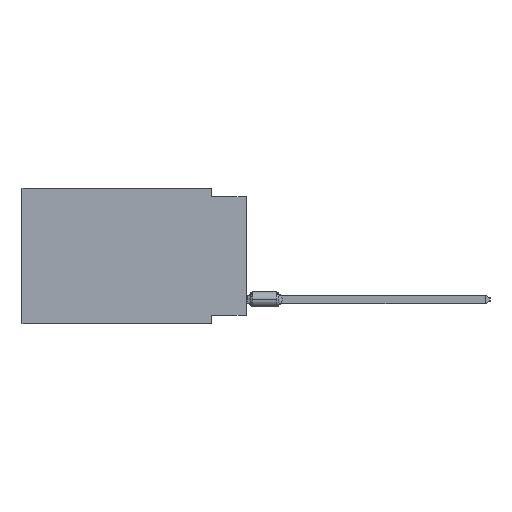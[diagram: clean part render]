
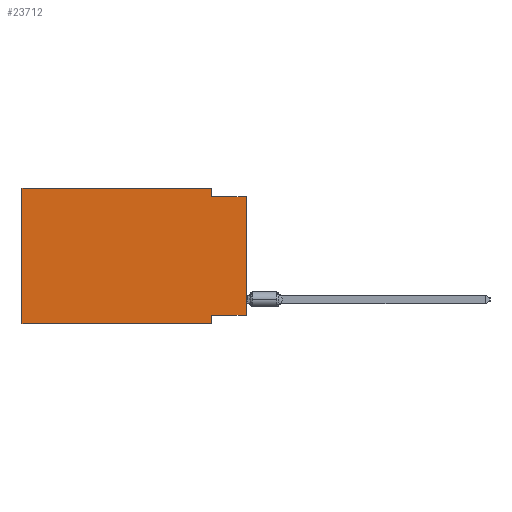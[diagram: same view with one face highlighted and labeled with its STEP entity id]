
A CAD part, left-side view. The second image highlights one B-rep face of the part: STEP entity #23712.
In plain terms, the highlighted planar face has unit normal (-1, 0, 0).
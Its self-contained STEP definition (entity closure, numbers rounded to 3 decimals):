
#1113 = CARTESIAN_POINT ( 'NONE',  ( 0., 16.383, 0. ) ) ;
#2373 = CARTESIAN_POINT ( 'NONE',  ( 0., 2.54, -9.906 ) ) ;
#3141 = VECTOR ( 'NONE', #3512, 1000. ) ;
#3512 = DIRECTION ( 'NONE',  ( 0., 0., -1. ) ) ;
#3820 = CARTESIAN_POINT ( 'NONE',  ( 0., 16.383, 0. ) ) ;
#5066 = ORIENTED_EDGE ( 'NONE', *, *, #47466, .T. ) ;
#7582 = VERTEX_POINT ( 'NONE', #53721 ) ;
#8241 = ORIENTED_EDGE ( 'NONE', *, *, #48617, .F. ) ;
#8436 = VECTOR ( 'NONE', #38168, 1000. ) ;
#9163 = DIRECTION ( 'NONE',  ( 0., 0., -1. ) ) ;
#11869 = VECTOR ( 'NONE', #49822, 1000. ) ;
#12670 = EDGE_CURVE ( 'NONE', #59389, #61183, #68344, .T. ) ;
#13704 = DIRECTION ( 'NONE',  ( 1., 0., 0. ) ) ;
#14302 = CARTESIAN_POINT ( 'NONE',  ( 0., 2.54, -9.906 ) ) ;
#14385 = PLANE ( 'NONE',  #55197 ) ;
#15514 = CARTESIAN_POINT ( 'NONE',  ( 0., 0., -0.635 ) ) ;
#16459 = LINE ( 'NONE', #37714, #11869 ) ;
#16998 = DIRECTION ( 'NONE',  ( 0., -1., 0. ) ) ;
#17649 = VERTEX_POINT ( 'NONE', #27561 ) ;
#18275 = CARTESIAN_POINT ( 'NONE',  ( 0., 16.383, 0. ) ) ;
#19437 = VERTEX_POINT ( 'NONE', #59192 ) ;
#20833 = LINE ( 'NONE', #64769, #36791 ) ;
#22191 = ORIENTED_EDGE ( 'NONE', *, *, #49745, .T. ) ;
#22597 = EDGE_CURVE ( 'NONE', #62183, #17649, #51913, .T. ) ;
#23712 = ADVANCED_FACE ( 'NONE', ( #56230 ), #14385, .F. ) ;
#25051 = DIRECTION ( 'NONE',  ( 0., -1., 0. ) ) ;
#27561 = CARTESIAN_POINT ( 'NONE',  ( 0., 2.54, 0. ) ) ;
#31141 = EDGE_CURVE ( 'NONE', #7582, #59389, #46911, .T. ) ;
#34273 = ORIENTED_EDGE ( 'NONE', *, *, #31141, .F. ) ;
#34578 = EDGE_CURVE ( 'NONE', #19437, #63240, #20833, .T. ) ;
#34847 = VECTOR ( 'NONE', #57052, 1000. ) ;
#35035 = VECTOR ( 'NONE', #63828, 1000. ) ;
#35773 = CARTESIAN_POINT ( 'NONE',  ( 0., 0., -9.271 ) ) ;
#36288 = EDGE_LOOP ( 'NONE', ( #5066, #51795, #37182, #56428, #8241, #22191, #65856, #34273 ) ) ;
#36791 = VECTOR ( 'NONE', #16998, 1000. ) ;
#37182 = ORIENTED_EDGE ( 'NONE', *, *, #60316, .F. ) ;
#37714 = CARTESIAN_POINT ( 'NONE',  ( 0., 16.383, -9.906 ) ) ;
#38168 = DIRECTION ( 'NONE',  ( 0., 0., 1. ) ) ;
#40044 = CARTESIAN_POINT ( 'NONE',  ( 0., 16.383, -9.906 ) ) ;
#42195 = CARTESIAN_POINT ( 'NONE',  ( 0., 0., 0. ) ) ;
#46007 = CARTESIAN_POINT ( 'NONE',  ( 0., 2.54, -9.271 ) ) ;
#46092 = CARTESIAN_POINT ( 'NONE',  ( 0., 16.383, 0. ) ) ;
#46911 = LINE ( 'NONE', #35773, #34847 ) ;
#47466 = EDGE_CURVE ( 'NONE', #7582, #63240, #54041, .T. ) ;
#48617 = EDGE_CURVE ( 'NONE', #51685, #62183, #60466, .T. ) ;
#49745 = EDGE_CURVE ( 'NONE', #51685, #61183, #16459, .T. ) ;
#49822 = DIRECTION ( 'NONE',  ( 0., -1., 0. ) ) ;
#50675 = VECTOR ( 'NONE', #25051, 1000. ) ;
#51419 = LINE ( 'NONE', #61895, #66264 ) ;
#51685 = VERTEX_POINT ( 'NONE', #40044 ) ;
#51795 = ORIENTED_EDGE ( 'NONE', *, *, #34578, .F. ) ;
#51913 = LINE ( 'NONE', #3820, #50675 ) ;
#53721 = CARTESIAN_POINT ( 'NONE',  ( 0., 0., -9.271 ) ) ;
#54041 = LINE ( 'NONE', #42195, #35035 ) ;
#55197 = AXIS2_PLACEMENT_3D ( 'NONE', #46092, #13704, #9163 ) ;
#56230 = FACE_OUTER_BOUND ( 'NONE', #36288, .T. ) ;
#56428 = ORIENTED_EDGE ( 'NONE', *, *, #22597, .F. ) ;
#57052 = DIRECTION ( 'NONE',  ( 0., 1., 0. ) ) ;
#59192 = CARTESIAN_POINT ( 'NONE',  ( 0., 2.54, -0.635 ) ) ;
#59389 = VERTEX_POINT ( 'NONE', #46007 ) ;
#60316 = EDGE_CURVE ( 'NONE', #17649, #19437, #51419, .T. ) ;
#60466 = LINE ( 'NONE', #18275, #8436 ) ;
#61183 = VERTEX_POINT ( 'NONE', #2373 ) ;
#61895 = CARTESIAN_POINT ( 'NONE',  ( 0., 2.54, 0. ) ) ;
#62183 = VERTEX_POINT ( 'NONE', #1113 ) ;
#63240 = VERTEX_POINT ( 'NONE', #15514 ) ;
#63828 = DIRECTION ( 'NONE',  ( 0., 0., 1. ) ) ;
#64769 = CARTESIAN_POINT ( 'NONE',  ( 0., 0., -0.635 ) ) ;
#65856 = ORIENTED_EDGE ( 'NONE', *, *, #12670, .F. ) ;
#66264 = VECTOR ( 'NONE', #68517, 1000. ) ;
#68344 = LINE ( 'NONE', #14302, #3141 ) ;
#68517 = DIRECTION ( 'NONE',  ( 0., 0., -1. ) ) ;
